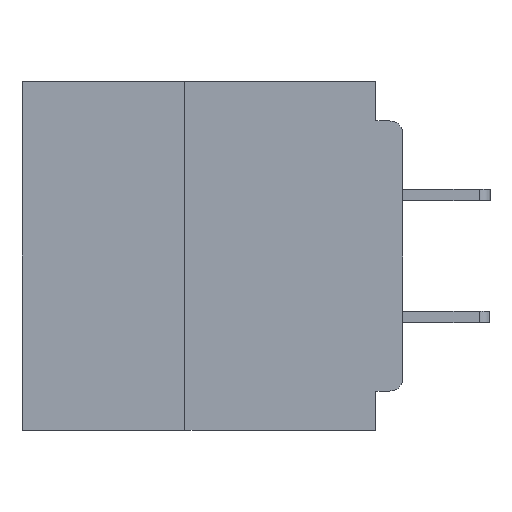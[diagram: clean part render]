
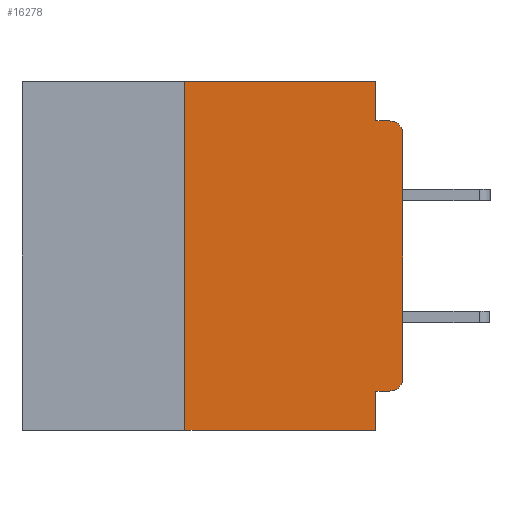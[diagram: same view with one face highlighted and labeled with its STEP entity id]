
A CAD part, left-side view. The second image highlights one B-rep face of the part: STEP entity #16278.
In plain terms, the highlighted planar face has unit normal (-1, 0, 0).
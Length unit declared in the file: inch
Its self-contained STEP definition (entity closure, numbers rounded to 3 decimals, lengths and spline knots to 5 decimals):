
#355 = ORIENTED_EDGE ( 'NONE', *, *, #7023, .F. ) ;
#396 = DIRECTION ( 'NONE',  ( 0., -1., 0. ) ) ;
#2134 = LINE ( 'NONE', #29421, #3211 ) ;
#2894 = EDGE_CURVE ( 'NONE', #13312, #8912, #29197, .T. ) ;
#3211 = VECTOR ( 'NONE', #8280, 39.37008 ) ;
#3459 = VECTOR ( 'NONE', #39909, 39.37008 ) ;
#4326 = AXIS2_PLACEMENT_3D ( 'NONE', #38497, #17481, #41971 ) ;
#4402 = CARTESIAN_POINT ( 'NONE',  ( 0., 0.015, -0.355 ) ) ;
#5299 = CARTESIAN_POINT ( 'NONE',  ( 0., 0.015, -0.045 ) ) ;
#6338 = VERTEX_POINT ( 'NONE', #37772 ) ;
#7023 = EDGE_CURVE ( 'NONE', #39187, #41984, #41804, .T. ) ;
#8280 = DIRECTION ( 'NONE',  ( 0., 0., -1. ) ) ;
#8390 = PLANE ( 'NONE',  #26691 ) ;
#8912 = VERTEX_POINT ( 'NONE', #5299 ) ;
#9636 = EDGE_CURVE ( 'NONE', #45274, #20717, #36208, .T. ) ;
#10059 = AXIS2_PLACEMENT_3D ( 'NONE', #32193, #11065, #35724 ) ;
#10585 = VECTOR ( 'NONE', #35452, 39.37008 ) ;
#11065 = DIRECTION ( 'NONE',  ( -1., 0., 0. ) ) ;
#12657 = VECTOR ( 'NONE', #396, 39.37008 ) ;
#12988 = CARTESIAN_POINT ( 'NONE',  ( 0., 0.25, -0.4 ) ) ;
#13312 = VERTEX_POINT ( 'NONE', #34459 ) ;
#13411 = VERTEX_POINT ( 'NONE', #24632 ) ;
#14369 = VERTEX_POINT ( 'NONE', #44186 ) ;
#15269 = ORIENTED_EDGE ( 'NONE', *, *, #23689, .F. ) ;
#16278 = ADVANCED_FACE ( 'NONE', ( #35717 ), #8390, .F. ) ;
#16985 = CARTESIAN_POINT ( 'NONE',  ( 0., 0.437, 0. ) ) ;
#16991 = EDGE_LOOP ( 'NONE', ( #44740, #19233, #30951, #36746, #355, #15269, #33221, #31760, #17783, #39587 ) ) ;
#17481 = DIRECTION ( 'NONE',  ( -1., 0., 0. ) ) ;
#17527 = VECTOR ( 'NONE', #27289, 39.37008 ) ;
#17783 = ORIENTED_EDGE ( 'NONE', *, *, #9636, .F. ) ;
#18896 = LINE ( 'NONE', #44545, #36454 ) ;
#19091 = CARTESIAN_POINT ( 'NONE',  ( 0., 0.437, 0. ) ) ;
#19233 = ORIENTED_EDGE ( 'NONE', *, *, #25644, .T. ) ;
#20038 = LINE ( 'NONE', #35141, #10585 ) ;
#20231 = CARTESIAN_POINT ( 'NONE',  ( 0., 0., -0.355 ) ) ;
#20542 = DIRECTION ( 'NONE',  ( 0., -1., 0. ) ) ;
#20717 = VERTEX_POINT ( 'NONE', #21714 ) ;
#21197 = LINE ( 'NONE', #22321, #3459 ) ;
#21204 = CARTESIAN_POINT ( 'NONE',  ( 0., 0.031, 0. ) ) ;
#21218 = EDGE_CURVE ( 'NONE', #45274, #6338, #31317, .T. ) ;
#21714 = CARTESIAN_POINT ( 'NONE',  ( 0., 0.031, -0.355 ) ) ;
#22092 = CIRCLE ( 'NONE', #10059, 0.015 ) ;
#22321 = CARTESIAN_POINT ( 'NONE',  ( 0., 0., 0. ) ) ;
#22648 = DIRECTION ( 'NONE',  ( 0., 0., -1. ) ) ;
#23227 = VECTOR ( 'NONE', #20542, 39.37008 ) ;
#23689 = EDGE_CURVE ( 'NONE', #13411, #39187, #37546, .T. ) ;
#24632 = CARTESIAN_POINT ( 'NONE',  ( 0., 0.25, -0.4 ) ) ;
#25644 = EDGE_CURVE ( 'NONE', #14369, #8912, #22092, .T. ) ;
#26691 = AXIS2_PLACEMENT_3D ( 'NONE', #19091, #43569, #22648 ) ;
#27289 = DIRECTION ( 'NONE',  ( 0., 1., 0. ) ) ;
#27427 = DIRECTION ( 'NONE',  ( 0., -1., 0. ) ) ;
#29197 = LINE ( 'NONE', #42516, #12657 ) ;
#29421 = CARTESIAN_POINT ( 'NONE',  ( 0., 0.031, -0.4 ) ) ;
#30951 = ORIENTED_EDGE ( 'NONE', *, *, #2894, .F. ) ;
#31317 = CIRCLE ( 'NONE', #4326, 0.015 ) ;
#31760 = ORIENTED_EDGE ( 'NONE', *, *, #33852, .F. ) ;
#32193 = CARTESIAN_POINT ( 'NONE',  ( 0., 0.015, -0.06 ) ) ;
#33221 = ORIENTED_EDGE ( 'NONE', *, *, #42495, .T. ) ;
#33852 = EDGE_CURVE ( 'NONE', #20717, #38380, #2134, .T. ) ;
#34459 = CARTESIAN_POINT ( 'NONE',  ( 0., 0.031, -0.045 ) ) ;
#35141 = CARTESIAN_POINT ( 'NONE',  ( 0., 0.031, 0. ) ) ;
#35350 = VECTOR ( 'NONE', #44599, 39.37008 ) ;
#35452 = DIRECTION ( 'NONE',  ( 0., 0., -1. ) ) ;
#35717 = FACE_OUTER_BOUND ( 'NONE', #16991, .T. ) ;
#35724 = DIRECTION ( 'NONE',  ( 0., 0., -1. ) ) ;
#36208 = LINE ( 'NONE', #20231, #17527 ) ;
#36454 = VECTOR ( 'NONE', #27427, 39.37008 ) ;
#36746 = ORIENTED_EDGE ( 'NONE', *, *, #42020, .F. ) ;
#37546 = LINE ( 'NONE', #12988, #35350 ) ;
#37772 = CARTESIAN_POINT ( 'NONE',  ( 0., 0., -0.34 ) ) ;
#38380 = VERTEX_POINT ( 'NONE', #44441 ) ;
#38497 = CARTESIAN_POINT ( 'NONE',  ( 0., 0.015, -0.34 ) ) ;
#38780 = CARTESIAN_POINT ( 'NONE',  ( 0., 0.25, 0. ) ) ;
#39187 = VERTEX_POINT ( 'NONE', #38780 ) ;
#39587 = ORIENTED_EDGE ( 'NONE', *, *, #21218, .T. ) ;
#39909 = DIRECTION ( 'NONE',  ( 0., 0., 1. ) ) ;
#41560 = EDGE_CURVE ( 'NONE', #6338, #14369, #21197, .T. ) ;
#41804 = LINE ( 'NONE', #16985, #23227 ) ;
#41971 = DIRECTION ( 'NONE',  ( 0., 0., -1. ) ) ;
#41984 = VERTEX_POINT ( 'NONE', #21204 ) ;
#42020 = EDGE_CURVE ( 'NONE', #41984, #13312, #20038, .T. ) ;
#42495 = EDGE_CURVE ( 'NONE', #13411, #38380, #18896, .T. ) ;
#42516 = CARTESIAN_POINT ( 'NONE',  ( 0., 0., -0.045 ) ) ;
#43569 = DIRECTION ( 'NONE',  ( 1., 0., 0. ) ) ;
#44186 = CARTESIAN_POINT ( 'NONE',  ( 0., 0., -0.06 ) ) ;
#44441 = CARTESIAN_POINT ( 'NONE',  ( 0., 0.031, -0.4 ) ) ;
#44545 = CARTESIAN_POINT ( 'NONE',  ( 0., 0.437, -0.4 ) ) ;
#44599 = DIRECTION ( 'NONE',  ( 0., 0., 1. ) ) ;
#44740 = ORIENTED_EDGE ( 'NONE', *, *, #41560, .T. ) ;
#45274 = VERTEX_POINT ( 'NONE', #4402 ) ;
